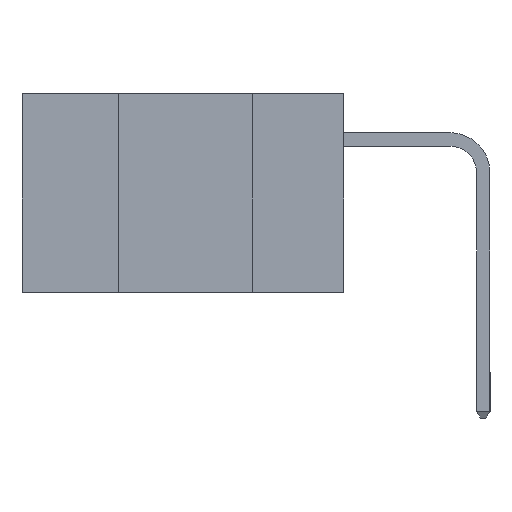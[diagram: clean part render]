
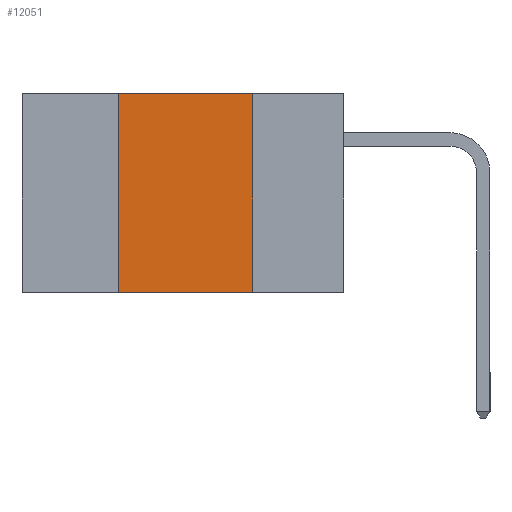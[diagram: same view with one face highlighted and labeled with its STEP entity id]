
A CAD part, left-side view. The second image highlights one B-rep face of the part: STEP entity #12051.
In plain terms, the highlighted planar face has unit normal (-1, 0, 0).
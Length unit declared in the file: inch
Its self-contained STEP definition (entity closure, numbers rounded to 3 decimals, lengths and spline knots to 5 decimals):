
#168 = ORIENTED_EDGE ( 'NONE', *, *, #10821, .F. ) ;
#890 = CARTESIAN_POINT ( 'NONE',  ( 0., 0.42, -0.37 ) ) ;
#1071 = VECTOR ( 'NONE', #14592, 39.37008 ) ;
#1257 = FACE_OUTER_BOUND ( 'NONE', #12334, .T. ) ;
#1445 = CARTESIAN_POINT ( 'NONE',  ( 0., 0.17, 0. ) ) ;
#1904 = VERTEX_POINT ( 'NONE', #3249 ) ;
#2258 = DIRECTION ( 'NONE',  ( 0., -1., 0. ) ) ;
#2579 = LINE ( 'NONE', #13438, #14134 ) ;
#2746 = VERTEX_POINT ( 'NONE', #6791 ) ;
#2907 = VERTEX_POINT ( 'NONE', #3212 ) ;
#3212 = CARTESIAN_POINT ( 'NONE',  ( 0., 0.42, 0. ) ) ;
#3249 = CARTESIAN_POINT ( 'NONE',  ( 0., 0.42, -0.37 ) ) ;
#3293 = CARTESIAN_POINT ( 'NONE',  ( 0., 0.6, -0.37 ) ) ;
#3965 = ORIENTED_EDGE ( 'NONE', *, *, #9855, .F. ) ;
#4639 = DIRECTION ( 'NONE',  ( 0., 0., 1. ) ) ;
#4678 = LINE ( 'NONE', #12264, #1071 ) ;
#4908 = EDGE_CURVE ( 'NONE', #1904, #2746, #13194, .T. ) ;
#4927 = CARTESIAN_POINT ( 'NONE',  ( 0., 0.6, 0. ) ) ;
#6221 = ORIENTED_EDGE ( 'NONE', *, *, #4908, .T. ) ;
#6791 = CARTESIAN_POINT ( 'NONE',  ( 0., 0.17, -0.37 ) ) ;
#8789 = DIRECTION ( 'NONE',  ( 0., 0., -1. ) ) ;
#9799 = DIRECTION ( 'NONE',  ( 0., 0., -1. ) ) ;
#9855 = EDGE_CURVE ( 'NONE', #1904, #2907, #10547, .T. ) ;
#10470 = AXIS2_PLACEMENT_3D ( 'NONE', #4927, #11242, #9799 ) ;
#10536 = ORIENTED_EDGE ( 'NONE', *, *, #14767, .F. ) ;
#10547 = LINE ( 'NONE', #890, #14329 ) ;
#10821 = EDGE_CURVE ( 'NONE', #2907, #11377, #4678, .T. ) ;
#11009 = PLANE ( 'NONE',  #10470 ) ;
#11242 = DIRECTION ( 'NONE',  ( 1., 0., 0. ) ) ;
#11377 = VERTEX_POINT ( 'NONE', #1445 ) ;
#11431 = VECTOR ( 'NONE', #2258, 39.37008 ) ;
#12051 = ADVANCED_FACE ( 'NONE', ( #1257 ), #11009, .F. ) ;
#12264 = CARTESIAN_POINT ( 'NONE',  ( 0., 0.6, 0. ) ) ;
#12334 = EDGE_LOOP ( 'NONE', ( #10536, #168, #3965, #6221 ) ) ;
#13194 = LINE ( 'NONE', #3293, #11431 ) ;
#13438 = CARTESIAN_POINT ( 'NONE',  ( 0., 0.17, -0.37 ) ) ;
#14134 = VECTOR ( 'NONE', #8789, 39.37008 ) ;
#14329 = VECTOR ( 'NONE', #4639, 39.37008 ) ;
#14592 = DIRECTION ( 'NONE',  ( 0., -1., 0. ) ) ;
#14767 = EDGE_CURVE ( 'NONE', #11377, #2746, #2579, .T. ) ;
